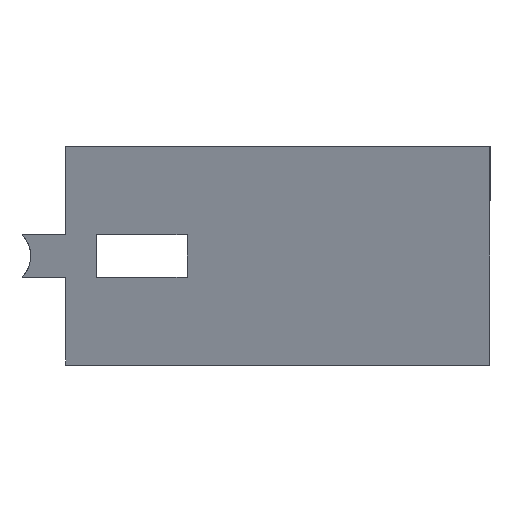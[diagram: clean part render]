
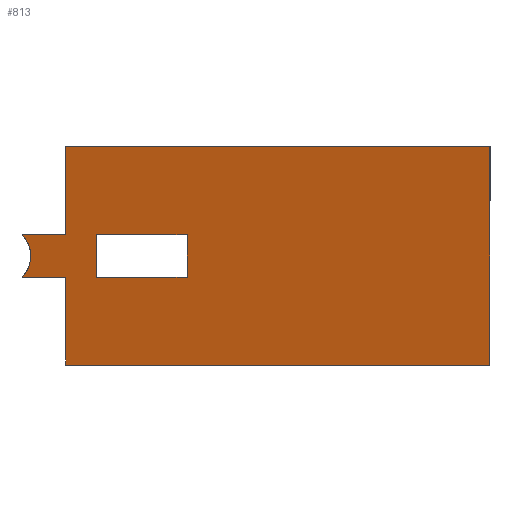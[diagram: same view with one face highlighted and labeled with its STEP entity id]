
A CAD part, left-side view. The second image highlights one B-rep face of the part: STEP entity #813.
In plain terms, the highlighted planar face has unit normal (-0.94, 0.342, 0).
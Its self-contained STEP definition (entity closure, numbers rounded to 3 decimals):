
#17 = ORIENTED_EDGE ( 'NONE', *, *, #1248, .T. ) ;
#18 = EDGE_CURVE ( 'NONE', #664, #1147, #1721, .T. ) ;
#37 = CARTESIAN_POINT ( 'NONE',  ( -40.91, -10., 0. ) ) ;
#47 = CARTESIAN_POINT ( 'NONE',  ( -52.728, -42.47, -7.25 ) ) ;
#60 = ORIENTED_EDGE ( 'NONE', *, *, #983, .F. ) ;
#65 = CARTESIAN_POINT ( 'NONE',  ( -47.279, -27.5, 10.75 ) ) ;
#78 = CARTESIAN_POINT ( 'NONE',  ( -47.279, -27.5, -7.25 ) ) ;
#120 = CARTESIAN_POINT ( 'NONE',  ( -38.68, -3.873, 3.5 ) ) ;
#125 = DIRECTION ( 'NONE',  ( 0., 0., 1. ) ) ;
#157 = CARTESIAN_POINT ( 'NONE',  ( -43.64, -17.5, 3.5 ) ) ;
#173 = EDGE_CURVE ( 'NONE', #1710, #318, #2105, .T. ) ;
#183 = LINE ( 'NONE', #1204, #1453 ) ;
#187 = CARTESIAN_POINT ( 'NONE',  ( -40., -7.5, 10.75 ) ) ;
#211 = CARTESIAN_POINT ( 'NONE',  ( -32.91, 11.978, 3.5 ) ) ;
#222 = ORIENTED_EDGE ( 'NONE', *, *, #173, .T. ) ;
#225 = CARTESIAN_POINT ( 'NONE',  ( -40.91, -10., 10.75 ) ) ;
#232 = DIRECTION ( 'NONE',  ( 0., 0., -1. ) ) ;
#249 = DIRECTION ( 'NONE',  ( -0.342, -0.94, 0. ) ) ;
#252 = CARTESIAN_POINT ( 'NONE',  ( -47.279, -27.5, 10.75 ) ) ;
#260 = DIRECTION ( 'NONE',  ( 0.342, 0.94, 0. ) ) ;
#318 = VERTEX_POINT ( 'NONE', #1354 ) ;
#375 = CARTESIAN_POINT ( 'NONE',  ( -47.279, -27.5, 0. ) ) ;
#390 = ORIENTED_EDGE ( 'NONE', *, *, #1795, .F. ) ;
#399 = CARTESIAN_POINT ( 'NONE',  ( -40., -7.5, 3.5 ) ) ;
#405 = EDGE_CURVE ( 'NONE', #664, #673, #587, .T. ) ;
#504 = VERTEX_POINT ( 'NONE', #157 ) ;
#515 = VECTOR ( 'NONE', #232, 1000. ) ;
#540 = VECTOR ( 'NONE', #1668, 1000. ) ;
#544 = CARTESIAN_POINT ( 'NONE',  ( -43.64, -17.5, 0. ) ) ;
#552 = ORIENTED_EDGE ( 'NONE', *, *, #1427, .F. ) ;
#562 = CARTESIAN_POINT ( 'NONE',  ( -40., -7.5, 0. ) ) ;
#568 = DIRECTION ( 'NONE',  ( 0.342, 0.94, 0. ) ) ;
#585 = FACE_BOUND ( 'NONE', #908, .T. ) ;
#587 = LINE ( 'NONE', #1882, #978 ) ;
#620 = VERTEX_POINT ( 'NONE', #1286 ) ;
#631 = LINE ( 'NONE', #821, #968 ) ;
#664 = VERTEX_POINT ( 'NONE', #731 ) ;
#673 = VERTEX_POINT ( 'NONE', #47 ) ;
#682 = ORIENTED_EDGE ( 'NONE', *, *, #1028, .F. ) ;
#731 = CARTESIAN_POINT ( 'NONE',  ( -52.728, -42.47, 10.75 ) ) ;
#740 = ORIENTED_EDGE ( 'NONE', *, *, #405, .F. ) ;
#811 = CARTESIAN_POINT ( 'NONE',  ( -39.053, -4.898, 1.025 ) ) ;
#813 = ADVANCED_FACE ( 'NONE', ( #1181, #585 ), #1079, .T. ) ;
#821 = CARTESIAN_POINT ( 'NONE',  ( -43.64, -17.5, 10.75 ) ) ;
#850 = VERTEX_POINT ( 'NONE', #2030 ) ;
#877 = CARTESIAN_POINT ( 'NONE',  ( -47.279, -27.5, 3.5 ) ) ;
#883 = VECTOR ( 'NONE', #1881, 1000. ) ;
#884 = VECTOR ( 'NONE', #568, 1000. ) ;
#908 = EDGE_LOOP ( 'NONE', ( #390, #17, #682, #552 ) ) ;
#968 = VECTOR ( 'NONE', #125, 1000. ) ;
#974 = ORIENTED_EDGE ( 'NONE', *, *, #1571, .F. ) ;
#978 = VECTOR ( 'NONE', #2050, 1000. ) ;
#983 = EDGE_CURVE ( 'NONE', #1213, #620, #1878, .T. ) ;
#1028 = EDGE_CURVE ( 'NONE', #1432, #504, #631, .T. ) ;
#1035 = LINE ( 'NONE', #375, #540 ) ;
#1057 = CARTESIAN_POINT ( 'NONE',  ( -32.91, 11.978, 0. ) ) ;
#1069 = EDGE_LOOP ( 'NONE', ( #60, #974, #222, #1134, #740, #1583, #1984, #1630 ) ) ;
#1079 = PLANE ( 'NONE',  #1346 ) ;
#1134 = ORIENTED_EDGE ( 'NONE', *, *, #1922, .F. ) ;
#1143 = CARTESIAN_POINT ( 'NONE',  ( -39.053, -4.898, 2.475 ) ) ;
#1147 = VERTEX_POINT ( 'NONE', #1158 ) ;
#1158 = CARTESIAN_POINT ( 'NONE',  ( -40., -7.5, 10.75 ) ) ;
#1181 = FACE_OUTER_BOUND ( 'NONE', #1069, .T. ) ;
#1195 = LINE ( 'NONE', #877, #2008 ) ;
#1198 = DIRECTION ( 'NONE',  ( -0.342, -0.94, 0. ) ) ;
#1204 = CARTESIAN_POINT ( 'NONE',  ( -40., -7.5, 10.75 ) ) ;
#1213 = VERTEX_POINT ( 'NONE', #1330 ) ;
#1226 = DIRECTION ( 'NONE',  ( 0.342, 0.94, 0. ) ) ;
#1234 = DIRECTION ( 'NONE',  ( 0., 0., -1. ) ) ;
#1248 = EDGE_CURVE ( 'NONE', #850, #504, #1195, .T. ) ;
#1259 = DIRECTION ( 'NONE',  ( -0.94, 0.342, 0. ) ) ;
#1286 = CARTESIAN_POINT ( 'NONE',  ( -38.68, -3.873, 3.5 ) ) ;
#1311 = LINE ( 'NONE', #211, #884 ) ;
#1330 = CARTESIAN_POINT ( 'NONE',  ( -38.68, -3.873, 0. ) ) ;
#1346 = AXIS2_PLACEMENT_3D ( 'NONE', #65, #1259, #249 ) ;
#1354 = CARTESIAN_POINT ( 'NONE',  ( -40., -7.5, -7.25 ) ) ;
#1367 = EDGE_CURVE ( 'NONE', #1147, #1731, #183, .T. ) ;
#1427 = EDGE_CURVE ( 'NONE', #1602, #1432, #1035, .T. ) ;
#1432 = VERTEX_POINT ( 'NONE', #544 ) ;
#1453 = VECTOR ( 'NONE', #1661, 1000. ) ;
#1571 = EDGE_CURVE ( 'NONE', #1710, #1213, #1766, .T. ) ;
#1583 = ORIENTED_EDGE ( 'NONE', *, *, #18, .T. ) ;
#1602 = VERTEX_POINT ( 'NONE', #37 ) ;
#1605 = EDGE_CURVE ( 'NONE', #1731, #620, #1311, .T. ) ;
#1630 = ORIENTED_EDGE ( 'NONE', *, *, #1605, .T. ) ;
#1646 = VECTOR ( 'NONE', #260, 1000. ) ;
#1661 = DIRECTION ( 'NONE',  ( 0., 0., -1. ) ) ;
#1668 = DIRECTION ( 'NONE',  ( -0.342, -0.94, 0. ) ) ;
#1710 = VERTEX_POINT ( 'NONE', #562 ) ;
#1721 = LINE ( 'NONE', #252, #883 ) ;
#1722 = VECTOR ( 'NONE', #1226, 1000. ) ;
#1731 = VERTEX_POINT ( 'NONE', #399 ) ;
#1766 = LINE ( 'NONE', #1057, #1722 ) ;
#1795 = EDGE_CURVE ( 'NONE', #850, #1602, #1974, .T. ) ;
#1878 =( BOUNDED_CURVE ( )  B_SPLINE_CURVE ( 3, ( #1907, #811, #1143, #120 ),
 .UNSPECIFIED., .F., .T. ) 
 B_SPLINE_CURVE_WITH_KNOTS ( ( 4, 4 ),
 ( 2.356, 3.927 ),
 .UNSPECIFIED. ) 
 CURVE ( )  GEOMETRIC_REPRESENTATION_ITEM ( )  RATIONAL_B_SPLINE_CURVE ( ( 1., 0.805, 0.805, 1. ) ) 
 REPRESENTATION_ITEM ( '' )  );
#1881 = DIRECTION ( 'NONE',  ( 0.342, 0.94, 0. ) ) ;
#1882 = CARTESIAN_POINT ( 'NONE',  ( -52.728, -42.47, 10.75 ) ) ;
#1907 = CARTESIAN_POINT ( 'NONE',  ( -38.68, -3.873, 0. ) ) ;
#1922 = EDGE_CURVE ( 'NONE', #673, #318, #2058, .T. ) ;
#1974 = LINE ( 'NONE', #225, #2079 ) ;
#1984 = ORIENTED_EDGE ( 'NONE', *, *, #1367, .T. ) ;
#2008 = VECTOR ( 'NONE', #1198, 1000. ) ;
#2030 = CARTESIAN_POINT ( 'NONE',  ( -40.91, -10., 3.5 ) ) ;
#2050 = DIRECTION ( 'NONE',  ( 0., 0., -1. ) ) ;
#2058 = LINE ( 'NONE', #78, #1646 ) ;
#2079 = VECTOR ( 'NONE', #1234, 1000. ) ;
#2105 = LINE ( 'NONE', #187, #515 ) ;
